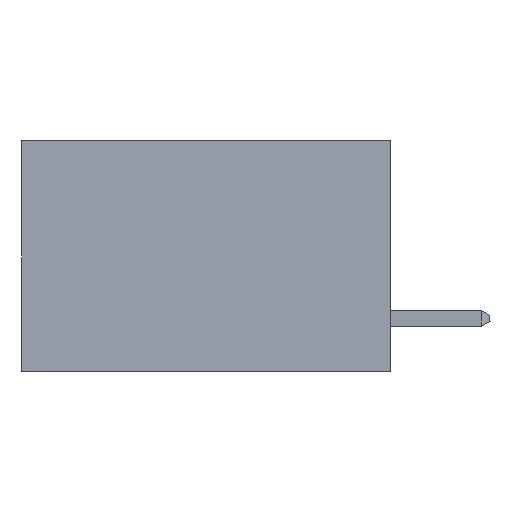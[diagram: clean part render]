
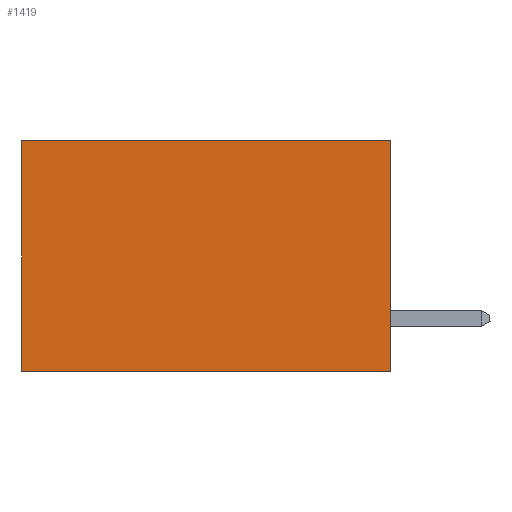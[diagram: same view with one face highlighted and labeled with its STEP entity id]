
A CAD part, left-side view. The second image highlights one B-rep face of the part: STEP entity #1419.
In plain terms, the highlighted planar face has unit normal (-1, 0, 0).
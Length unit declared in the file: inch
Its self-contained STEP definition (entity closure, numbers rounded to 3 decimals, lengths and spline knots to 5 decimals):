
#88 = ORIENTED_EDGE ( 'NONE', *, *, #4406, .F. ) ;
#390 = LINE ( 'NONE', #7498, #8238 ) ;
#759 = DIRECTION ( 'NONE',  ( 0., 1., 0. ) ) ;
#770 = FACE_OUTER_BOUND ( 'NONE', #890, .T. ) ;
#890 = EDGE_LOOP ( 'NONE', ( #10330, #88, #3929, #2261 ) ) ;
#919 = CARTESIAN_POINT ( 'NONE',  ( 0.277, 0.59, 0. ) ) ;
#1419 = ADVANCED_FACE ( 'NONE', ( #770 ), #9344, .F. ) ;
#1523 = DIRECTION ( 'NONE',  ( 0., 0., -1. ) ) ;
#1540 = VERTEX_POINT ( 'NONE', #12702 ) ;
#1573 = VECTOR ( 'NONE', #9839, 39.37008 ) ;
#2064 = CARTESIAN_POINT ( 'NONE',  ( 0.277, 0.59, -0.37 ) ) ;
#2098 = CARTESIAN_POINT ( 'NONE',  ( 0.277, 0., -0.37 ) ) ;
#2261 = ORIENTED_EDGE ( 'NONE', *, *, #9556, .T. ) ;
#2477 = EDGE_CURVE ( 'NONE', #6327, #10573, #6762, .T. ) ;
#3117 = DIRECTION ( 'NONE',  ( 0., 1., 0. ) ) ;
#3696 = VECTOR ( 'NONE', #3117, 39.37008 ) ;
#3929 = ORIENTED_EDGE ( 'NONE', *, *, #11517, .F. ) ;
#4406 = EDGE_CURVE ( 'NONE', #7980, #10573, #9864, .T. ) ;
#6305 = CARTESIAN_POINT ( 'NONE',  ( 0.277, 0., -0.37 ) ) ;
#6327 = VERTEX_POINT ( 'NONE', #919 ) ;
#6720 = LINE ( 'NONE', #7167, #3696 ) ;
#6762 = LINE ( 'NONE', #2064, #1573 ) ;
#7007 = CARTESIAN_POINT ( 'NONE',  ( 0.277, 0.59, -0.37 ) ) ;
#7167 = CARTESIAN_POINT ( 'NONE',  ( 0.277, 0., 0. ) ) ;
#7498 = CARTESIAN_POINT ( 'NONE',  ( 0.277, 0., -0.37 ) ) ;
#7980 = VERTEX_POINT ( 'NONE', #6305 ) ;
#8070 = CARTESIAN_POINT ( 'NONE',  ( 0.277, 0., -0.37 ) ) ;
#8238 = VECTOR ( 'NONE', #8450, 39.37008 ) ;
#8450 = DIRECTION ( 'NONE',  ( 0., 0., -1. ) ) ;
#9331 = DIRECTION ( 'NONE',  ( 1., 0., 0. ) ) ;
#9344 = PLANE ( 'NONE',  #10122 ) ;
#9556 = EDGE_CURVE ( 'NONE', #1540, #6327, #6720, .T. ) ;
#9839 = DIRECTION ( 'NONE',  ( 0., 0., -1. ) ) ;
#9864 = LINE ( 'NONE', #2098, #11736 ) ;
#10122 = AXIS2_PLACEMENT_3D ( 'NONE', #8070, #9331, #1523 ) ;
#10330 = ORIENTED_EDGE ( 'NONE', *, *, #2477, .T. ) ;
#10573 = VERTEX_POINT ( 'NONE', #7007 ) ;
#11517 = EDGE_CURVE ( 'NONE', #1540, #7980, #390, .T. ) ;
#11736 = VECTOR ( 'NONE', #759, 39.37008 ) ;
#12702 = CARTESIAN_POINT ( 'NONE',  ( 0.277, 0., 0. ) ) ;
